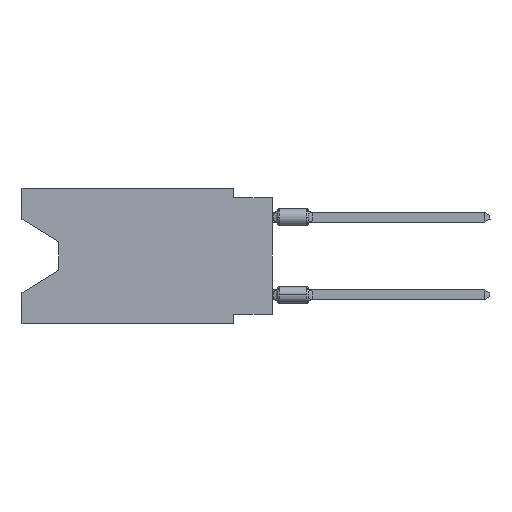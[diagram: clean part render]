
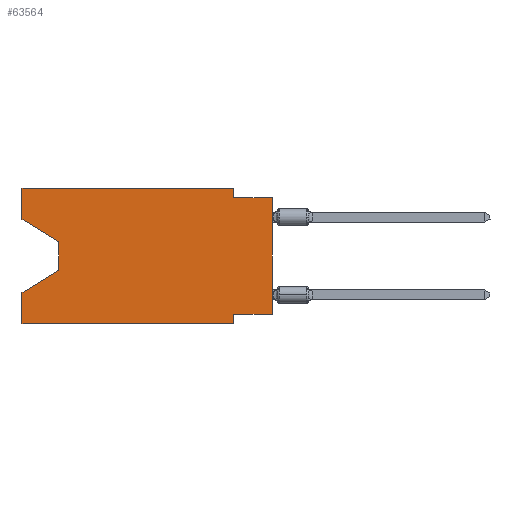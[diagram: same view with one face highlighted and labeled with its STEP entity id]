
A CAD part, left-side view. The second image highlights one B-rep face of the part: STEP entity #63564.
In plain terms, the highlighted planar face has unit normal (-1, 0, 0).
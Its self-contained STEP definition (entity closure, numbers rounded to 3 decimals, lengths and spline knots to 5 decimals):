
#470 = DIRECTION ( 'NONE',  ( 0., 0., -1. ) ) ;
#584 = ORIENTED_EDGE ( 'NONE', *, *, #35166, .F. ) ;
#605 = LINE ( 'NONE', #33432, #16913 ) ;
#1151 = VECTOR ( 'NONE', #59355, 39.37008 ) ;
#1405 = ORIENTED_EDGE ( 'NONE', *, *, #26349, .F. ) ;
#2823 = CARTESIAN_POINT ( 'NONE',  ( 0., 0.55, -0.212 ) ) ;
#2924 = EDGE_CURVE ( 'NONE', #44573, #44871, #13659, .T. ) ;
#3584 = EDGE_CURVE ( 'NONE', #44573, #49099, #33172, .T. ) ;
#3877 = CARTESIAN_POINT ( 'NONE',  ( 0., 0.645, -0.08025 ) ) ;
#4554 = ORIENTED_EDGE ( 'NONE', *, *, #59149, .F. ) ;
#4734 = CARTESIAN_POINT ( 'NONE',  ( 0., 0.1, -0.325 ) ) ;
#4872 = CARTESIAN_POINT ( 'NONE',  ( 0., 0.645, 0. ) ) ;
#5200 = LINE ( 'NONE', #17585, #10697 ) ;
#5626 = EDGE_CURVE ( 'NONE', #32303, #34006, #25365, .T. ) ;
#5790 = EDGE_CURVE ( 'NONE', #48995, #44871, #60407, .T. ) ;
#5913 = CARTESIAN_POINT ( 'NONE',  ( 0., 0., -0.025 ) ) ;
#6167 = VERTEX_POINT ( 'NONE', #71243 ) ;
#6203 = DIRECTION ( 'NONE',  ( 0., 1., 0. ) ) ;
#6596 = VECTOR ( 'NONE', #49745, 39.37008 ) ;
#7302 = CARTESIAN_POINT ( 'NONE',  ( 0., 0.55, -0.212 ) ) ;
#8842 = VERTEX_POINT ( 'NONE', #33337 ) ;
#9248 = DIRECTION ( 'NONE',  ( 0., 0., -1. ) ) ;
#9311 = DIRECTION ( 'NONE',  ( 0., 0., -1. ) ) ;
#9519 = VECTOR ( 'NONE', #55453, 39.37008 ) ;
#10697 = VECTOR ( 'NONE', #470, 39.37008 ) ;
#11302 = CARTESIAN_POINT ( 'NONE',  ( 0., 0., -0.325 ) ) ;
#11474 = ORIENTED_EDGE ( 'NONE', *, *, #5626, .T. ) ;
#13659 = LINE ( 'NONE', #64420, #42071 ) ;
#14117 = DIRECTION ( 'NONE',  ( 0., 0.855, -0.519 ) ) ;
#14386 = DIRECTION ( 'NONE',  ( 0., -1., 0. ) ) ;
#14934 = CARTESIAN_POINT ( 'NONE',  ( 0., 0., -0.325 ) ) ;
#15794 = LINE ( 'NONE', #60354, #6596 ) ;
#16637 = CARTESIAN_POINT ( 'NONE',  ( 0., 0.645, -0.35 ) ) ;
#16913 = VECTOR ( 'NONE', #34512, 39.37008 ) ;
#17074 = CARTESIAN_POINT ( 'NONE',  ( 0., 0.645, 0. ) ) ;
#17585 = CARTESIAN_POINT ( 'NONE',  ( 0., 0.1, 0. ) ) ;
#18081 = ORIENTED_EDGE ( 'NONE', *, *, #50511, .T. ) ;
#18206 = CARTESIAN_POINT ( 'NONE',  ( 0., 0.645, 0. ) ) ;
#18577 = EDGE_LOOP ( 'NONE', ( #23222, #48426, #18081, #59976, #37193, #40776, #4554, #11474, #1405, #584, #63907, #46161 ) ) ;
#23222 = ORIENTED_EDGE ( 'NONE', *, *, #68729, .T. ) ;
#24338 = VECTOR ( 'NONE', #9311, 39.37008 ) ;
#25183 = VERTEX_POINT ( 'NONE', #67232 ) ;
#25365 = LINE ( 'NONE', #69898, #40676 ) ;
#26349 = EDGE_CURVE ( 'NONE', #59395, #34006, #15794, .T. ) ;
#27385 = CARTESIAN_POINT ( 'NONE',  ( 0., 0.645, 0. ) ) ;
#27754 = LINE ( 'NONE', #11302, #44735 ) ;
#28377 = EDGE_CURVE ( 'NONE', #8842, #65511, #62783, .T. ) ;
#32303 = VERTEX_POINT ( 'NONE', #14934 ) ;
#33103 = DIRECTION ( 'NONE',  ( 0., -1., 0. ) ) ;
#33172 = LINE ( 'NONE', #17074, #9519 ) ;
#33337 = CARTESIAN_POINT ( 'NONE',  ( 0., 0.645, -0.08025 ) ) ;
#33432 = CARTESIAN_POINT ( 'NONE',  ( 0., 0.55, -0.138 ) ) ;
#34006 = VERTEX_POINT ( 'NONE', #5913 ) ;
#34313 = DIRECTION ( 'NONE',  ( 0., 0., 1. ) ) ;
#34512 = DIRECTION ( 'NONE',  ( 0., 0., -1. ) ) ;
#35166 = EDGE_CURVE ( 'NONE', #6167, #59395, #5200, .T. ) ;
#35671 = AXIS2_PLACEMENT_3D ( 'NONE', #4872, #59288, #9248 ) ;
#37193 = ORIENTED_EDGE ( 'NONE', *, *, #2924, .T. ) ;
#37449 = LINE ( 'NONE', #3877, #1151 ) ;
#38158 = EDGE_CURVE ( 'NONE', #65511, #6167, #61570, .T. ) ;
#40676 = VECTOR ( 'NONE', #68829, 39.37008 ) ;
#40776 = ORIENTED_EDGE ( 'NONE', *, *, #5790, .F. ) ;
#41594 = CARTESIAN_POINT ( 'NONE',  ( 0., 0.1, -0.025 ) ) ;
#42071 = VECTOR ( 'NONE', #14386, 39.37008 ) ;
#42742 = EDGE_CURVE ( 'NONE', #25183, #54659, #605, .T. ) ;
#43246 = CARTESIAN_POINT ( 'NONE',  ( 0., 0.1, -0.35 ) ) ;
#43352 = CARTESIAN_POINT ( 'NONE',  ( 0., 0.645, 0. ) ) ;
#44573 = VERTEX_POINT ( 'NONE', #16637 ) ;
#44735 = VECTOR ( 'NONE', #6203, 39.37008 ) ;
#44871 = VERTEX_POINT ( 'NONE', #43246 ) ;
#46161 = ORIENTED_EDGE ( 'NONE', *, *, #28377, .F. ) ;
#47965 = PLANE ( 'NONE',  #35671 ) ;
#48026 = CARTESIAN_POINT ( 'NONE',  ( 0., 0.1, -0.35 ) ) ;
#48426 = ORIENTED_EDGE ( 'NONE', *, *, #42742, .T. ) ;
#48995 = VERTEX_POINT ( 'NONE', #4734 ) ;
#49099 = VERTEX_POINT ( 'NONE', #57278 ) ;
#49745 = DIRECTION ( 'NONE',  ( 0., -1., 0. ) ) ;
#50511 = EDGE_CURVE ( 'NONE', #54659, #49099, #63422, .T. ) ;
#54659 = VERTEX_POINT ( 'NONE', #7302 ) ;
#55453 = DIRECTION ( 'NONE',  ( 0., 0., 1. ) ) ;
#57278 = CARTESIAN_POINT ( 'NONE',  ( 0., 0.645, -0.26975 ) ) ;
#57479 = VECTOR ( 'NONE', #33103, 39.37008 ) ;
#59149 = EDGE_CURVE ( 'NONE', #32303, #48995, #27754, .T. ) ;
#59288 = DIRECTION ( 'NONE',  ( 1., 0., 0. ) ) ;
#59355 = DIRECTION ( 'NONE',  ( 0., -0.855, -0.519 ) ) ;
#59395 = VERTEX_POINT ( 'NONE', #41594 ) ;
#59976 = ORIENTED_EDGE ( 'NONE', *, *, #3584, .F. ) ;
#60354 = CARTESIAN_POINT ( 'NONE',  ( 0., 0., -0.025 ) ) ;
#60407 = LINE ( 'NONE', #48026, #24338 ) ;
#61570 = LINE ( 'NONE', #43352, #57479 ) ;
#62783 = LINE ( 'NONE', #18206, #62799 ) ;
#62799 = VECTOR ( 'NONE', #34313, 39.37008 ) ;
#63422 = LINE ( 'NONE', #2823, #65213 ) ;
#63564 = ADVANCED_FACE ( 'NONE', ( #65092 ), #47965, .F. ) ;
#63907 = ORIENTED_EDGE ( 'NONE', *, *, #38158, .F. ) ;
#64420 = CARTESIAN_POINT ( 'NONE',  ( 0., 0.645, -0.35 ) ) ;
#65092 = FACE_OUTER_BOUND ( 'NONE', #18577, .T. ) ;
#65213 = VECTOR ( 'NONE', #14117, 39.37008 ) ;
#65511 = VERTEX_POINT ( 'NONE', #27385 ) ;
#67232 = CARTESIAN_POINT ( 'NONE',  ( 0., 0.55, -0.138 ) ) ;
#68729 = EDGE_CURVE ( 'NONE', #8842, #25183, #37449, .T. ) ;
#68829 = DIRECTION ( 'NONE',  ( 0., 0., 1. ) ) ;
#69898 = CARTESIAN_POINT ( 'NONE',  ( 0., 0., 0. ) ) ;
#71243 = CARTESIAN_POINT ( 'NONE',  ( 0., 0.1, 0. ) ) ;
